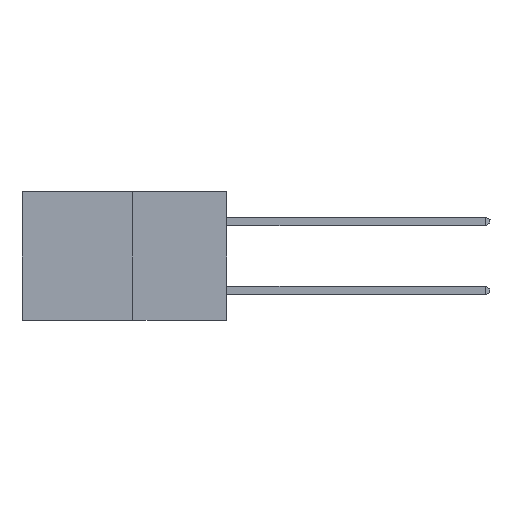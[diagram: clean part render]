
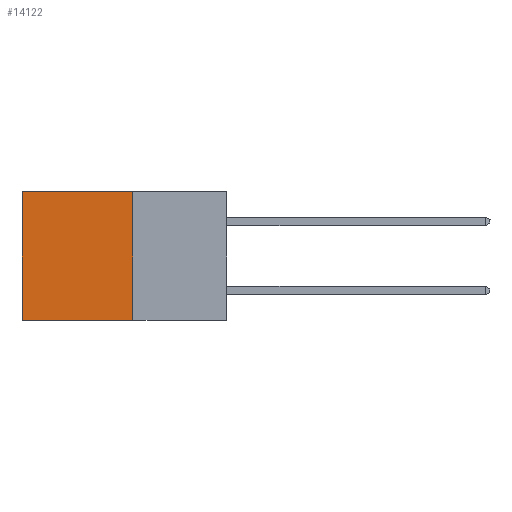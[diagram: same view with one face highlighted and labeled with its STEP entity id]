
A CAD part, left-side view. The second image highlights one B-rep face of the part: STEP entity #14122.
In plain terms, the highlighted planar face has unit normal (-1, 0, 0).
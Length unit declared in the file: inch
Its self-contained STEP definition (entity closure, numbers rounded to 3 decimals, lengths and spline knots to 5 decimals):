
#130 = VERTEX_POINT ( 'NONE', #20820 ) ;
#528 = CARTESIAN_POINT ( 'NONE',  ( 0.277, 0.27, -0.37 ) ) ;
#564 = DIRECTION ( 'NONE',  ( 0., 0., -1. ) ) ;
#1736 = PLANE ( 'NONE',  #14428 ) ;
#4221 = EDGE_CURVE ( 'NONE', #130, #6655, #23369, .T. ) ;
#5069 = CARTESIAN_POINT ( 'NONE',  ( 0.277, 0.59, -0.37 ) ) ;
#5718 = EDGE_LOOP ( 'NONE', ( #21456, #19871, #13126, #8419 ) ) ;
#6269 = EDGE_CURVE ( 'NONE', #6655, #6878, #13506, .T. ) ;
#6655 = VERTEX_POINT ( 'NONE', #22201 ) ;
#6664 = VERTEX_POINT ( 'NONE', #12145 ) ;
#6878 = VERTEX_POINT ( 'NONE', #13037 ) ;
#8018 = EDGE_CURVE ( 'NONE', #130, #6664, #16078, .T. ) ;
#8024 = VECTOR ( 'NONE', #13056, 39.37008 ) ;
#8419 = ORIENTED_EDGE ( 'NONE', *, *, #8018, .T. ) ;
#8925 = CARTESIAN_POINT ( 'NONE',  ( 0.277, 0.27, -0.37 ) ) ;
#10121 = DIRECTION ( 'NONE',  ( 1., 0., 0. ) ) ;
#12145 = CARTESIAN_POINT ( 'NONE',  ( 0.277, 0.59, 0. ) ) ;
#12363 = DIRECTION ( 'NONE',  ( 0., 1., 0. ) ) ;
#13037 = CARTESIAN_POINT ( 'NONE',  ( 0.277, 0.59, -0.37 ) ) ;
#13056 = DIRECTION ( 'NONE',  ( 0., 1., 0. ) ) ;
#13126 = ORIENTED_EDGE ( 'NONE', *, *, #4221, .F. ) ;
#13405 = DIRECTION ( 'NONE',  ( 0., 0., -1. ) ) ;
#13506 = LINE ( 'NONE', #8925, #8024 ) ;
#14122 = ADVANCED_FACE ( 'NONE', ( #25612 ), #1736, .F. ) ;
#14428 = AXIS2_PLACEMENT_3D ( 'NONE', #22247, #10121, #24252 ) ;
#16078 = LINE ( 'NONE', #24419, #16707 ) ;
#16707 = VECTOR ( 'NONE', #12363, 39.37008 ) ;
#18002 = VECTOR ( 'NONE', #564, 39.37008 ) ;
#18324 = EDGE_CURVE ( 'NONE', #6664, #6878, #26305, .T. ) ;
#19871 = ORIENTED_EDGE ( 'NONE', *, *, #6269, .F. ) ;
#20341 = VECTOR ( 'NONE', #13405, 39.37008 ) ;
#20820 = CARTESIAN_POINT ( 'NONE',  ( 0.277, 0.27, 0. ) ) ;
#21456 = ORIENTED_EDGE ( 'NONE', *, *, #18324, .T. ) ;
#22201 = CARTESIAN_POINT ( 'NONE',  ( 0.277, 0.27, -0.37 ) ) ;
#22247 = CARTESIAN_POINT ( 'NONE',  ( 0.277, 0.27, -0.37 ) ) ;
#23369 = LINE ( 'NONE', #528, #18002 ) ;
#24252 = DIRECTION ( 'NONE',  ( 0., 0., -1. ) ) ;
#24419 = CARTESIAN_POINT ( 'NONE',  ( 0.277, 0.27, 0. ) ) ;
#25612 = FACE_OUTER_BOUND ( 'NONE', #5718, .T. ) ;
#26305 = LINE ( 'NONE', #5069, #20341 ) ;
